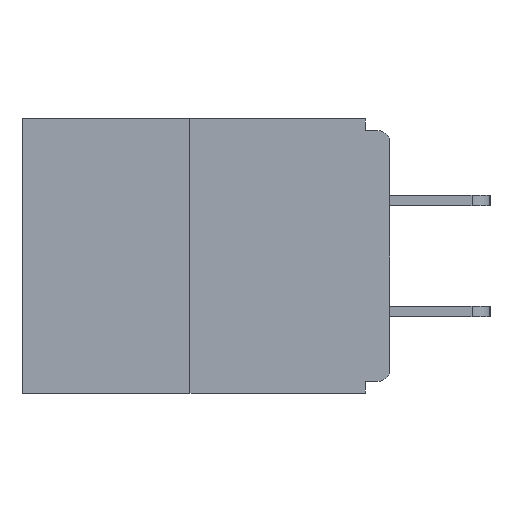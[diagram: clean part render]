
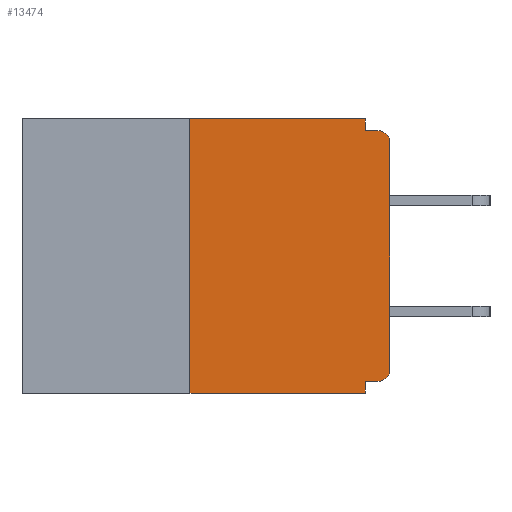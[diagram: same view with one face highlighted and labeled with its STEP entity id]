
A CAD part, left-side view. The second image highlights one B-rep face of the part: STEP entity #13474.
In plain terms, the highlighted planar face has unit normal (-1, 0, 0).
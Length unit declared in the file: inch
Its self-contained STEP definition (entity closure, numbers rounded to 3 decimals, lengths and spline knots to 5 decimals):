
#131 = CIRCLE ( 'NONE', #12091, 0.015 ) ;
#201 = VERTEX_POINT ( 'NONE', #5705 ) ;
#666 = DIRECTION ( 'NONE',  ( 0., 0., -1. ) ) ;
#750 = LINE ( 'NONE', #16430, #5694 ) ;
#1241 = CARTESIAN_POINT ( 'NONE',  ( 0., 0.031, 0. ) ) ;
#1309 = VECTOR ( 'NONE', #6027, 39.37008 ) ;
#1443 = CARTESIAN_POINT ( 'NONE',  ( 0., 0., -0.015 ) ) ;
#1554 = CARTESIAN_POINT ( 'NONE',  ( 0., 0.25, 0. ) ) ;
#1595 = ORIENTED_EDGE ( 'NONE', *, *, #3636, .F. ) ;
#1633 = EDGE_CURVE ( 'NONE', #12355, #9322, #1980, .T. ) ;
#1980 = CIRCLE ( 'NONE', #6410, 0.015 ) ;
#2694 = ORIENTED_EDGE ( 'NONE', *, *, #14655, .F. ) ;
#2749 = ORIENTED_EDGE ( 'NONE', *, *, #6295, .F. ) ;
#2947 = DIRECTION ( 'NONE',  ( 0., -1., 0. ) ) ;
#2991 = DIRECTION ( 'NONE',  ( 0., -1., 0. ) ) ;
#3419 = VERTEX_POINT ( 'NONE', #14173 ) ;
#3467 = EDGE_CURVE ( 'NONE', #9322, #201, #4333, .T. ) ;
#3636 = EDGE_CURVE ( 'NONE', #8145, #17130, #11496, .T. ) ;
#3654 = LINE ( 'NONE', #1443, #10410 ) ;
#4008 = VECTOR ( 'NONE', #2991, 39.37008 ) ;
#4129 = CARTESIAN_POINT ( 'NONE',  ( 0., 0.031, -0.015 ) ) ;
#4143 = ORIENTED_EDGE ( 'NONE', *, *, #8824, .F. ) ;
#4290 = DIRECTION ( 'NONE',  ( 0., 0., -1. ) ) ;
#4333 = LINE ( 'NONE', #5787, #8614 ) ;
#4971 = CARTESIAN_POINT ( 'NONE',  ( 0., 0.015, -0.313 ) ) ;
#5060 = CARTESIAN_POINT ( 'NONE',  ( 0., 0.015, -0.328 ) ) ;
#5574 = ORIENTED_EDGE ( 'NONE', *, *, #17512, .T. ) ;
#5694 = VECTOR ( 'NONE', #666, 39.37008 ) ;
#5705 = CARTESIAN_POINT ( 'NONE',  ( 0., 0., -0.03 ) ) ;
#5718 = VERTEX_POINT ( 'NONE', #4129 ) ;
#5787 = CARTESIAN_POINT ( 'NONE',  ( 0., 0., 0. ) ) ;
#6027 = DIRECTION ( 'NONE',  ( 0., -1., 0. ) ) ;
#6063 = CARTESIAN_POINT ( 'NONE',  ( 0., 0.25, 0. ) ) ;
#6295 = EDGE_CURVE ( 'NONE', #13297, #5718, #8324, .T. ) ;
#6410 = AXIS2_PLACEMENT_3D ( 'NONE', #4971, #13530, #13633 ) ;
#7028 = CARTESIAN_POINT ( 'NONE',  ( 0., 0.015, -0.03 ) ) ;
#7200 = VERTEX_POINT ( 'NONE', #14852 ) ;
#8093 = EDGE_CURVE ( 'NONE', #8145, #7200, #16721, .T. ) ;
#8145 = VERTEX_POINT ( 'NONE', #15782 ) ;
#8324 = LINE ( 'NONE', #1241, #17197 ) ;
#8614 = VECTOR ( 'NONE', #15790, 39.37008 ) ;
#8824 = EDGE_CURVE ( 'NONE', #17130, #13297, #17367, .T. ) ;
#8967 = CARTESIAN_POINT ( 'NONE',  ( 0., 0.015, -0.015 ) ) ;
#9135 = LINE ( 'NONE', #9775, #10214 ) ;
#9322 = VERTEX_POINT ( 'NONE', #10480 ) ;
#9775 = CARTESIAN_POINT ( 'NONE',  ( 0., 0., -0.328 ) ) ;
#10195 = CARTESIAN_POINT ( 'NONE',  ( 0., 0.46, 0. ) ) ;
#10214 = VECTOR ( 'NONE', #12315, 39.37008 ) ;
#10410 = VECTOR ( 'NONE', #2947, 39.37008 ) ;
#10480 = CARTESIAN_POINT ( 'NONE',  ( 0., 0., -0.313 ) ) ;
#10680 = DIRECTION ( 'NONE',  ( 1., 0., 0. ) ) ;
#10718 = ORIENTED_EDGE ( 'NONE', *, *, #8093, .T. ) ;
#10785 = DIRECTION ( 'NONE',  ( 0., 0., -1. ) ) ;
#11492 = CARTESIAN_POINT ( 'NONE',  ( 0., 0.46, -0.343 ) ) ;
#11496 = LINE ( 'NONE', #1554, #11742 ) ;
#11742 = VECTOR ( 'NONE', #11757, 39.37008 ) ;
#11757 = DIRECTION ( 'NONE',  ( 0., 0., 1. ) ) ;
#11811 = CARTESIAN_POINT ( 'NONE',  ( 0., 0.031, 0. ) ) ;
#12091 = AXIS2_PLACEMENT_3D ( 'NONE', #7028, #16963, #12701 ) ;
#12315 = DIRECTION ( 'NONE',  ( 0., 1., 0. ) ) ;
#12355 = VERTEX_POINT ( 'NONE', #5060 ) ;
#12701 = DIRECTION ( 'NONE',  ( 0., 0., -1. ) ) ;
#12763 = ORIENTED_EDGE ( 'NONE', *, *, #17640, .F. ) ;
#13059 = ORIENTED_EDGE ( 'NONE', *, *, #1633, .T. ) ;
#13297 = VERTEX_POINT ( 'NONE', #11811 ) ;
#13372 = VERTEX_POINT ( 'NONE', #8967 ) ;
#13474 = ADVANCED_FACE ( 'NONE', ( #13569 ), #15072, .F. ) ;
#13530 = DIRECTION ( 'NONE',  ( -1., 0., 0. ) ) ;
#13569 = FACE_OUTER_BOUND ( 'NONE', #15793, .T. ) ;
#13633 = DIRECTION ( 'NONE',  ( 0., 0., -1. ) ) ;
#14073 = ORIENTED_EDGE ( 'NONE', *, *, #18419, .F. ) ;
#14173 = CARTESIAN_POINT ( 'NONE',  ( 0., 0.031, -0.328 ) ) ;
#14655 = EDGE_CURVE ( 'NONE', #12355, #3419, #9135, .T. ) ;
#14852 = CARTESIAN_POINT ( 'NONE',  ( 0., 0.031, -0.343 ) ) ;
#14889 = AXIS2_PLACEMENT_3D ( 'NONE', #14951, #10680, #10785 ) ;
#14951 = CARTESIAN_POINT ( 'NONE',  ( 0., 0.46, 0. ) ) ;
#15072 = PLANE ( 'NONE',  #14889 ) ;
#15782 = CARTESIAN_POINT ( 'NONE',  ( 0., 0.25, -0.343 ) ) ;
#15790 = DIRECTION ( 'NONE',  ( 0., 0., 1. ) ) ;
#15793 = EDGE_LOOP ( 'NONE', ( #4143, #1595, #10718, #14073, #2694, #13059, #16270, #5574, #12763, #2749 ) ) ;
#16270 = ORIENTED_EDGE ( 'NONE', *, *, #3467, .T. ) ;
#16430 = CARTESIAN_POINT ( 'NONE',  ( 0., 0.031, -0.343 ) ) ;
#16721 = LINE ( 'NONE', #11492, #4008 ) ;
#16963 = DIRECTION ( 'NONE',  ( -1., 0., 0. ) ) ;
#17130 = VERTEX_POINT ( 'NONE', #6063 ) ;
#17197 = VECTOR ( 'NONE', #4290, 39.37008 ) ;
#17367 = LINE ( 'NONE', #10195, #1309 ) ;
#17512 = EDGE_CURVE ( 'NONE', #201, #13372, #131, .T. ) ;
#17640 = EDGE_CURVE ( 'NONE', #5718, #13372, #3654, .T. ) ;
#18419 = EDGE_CURVE ( 'NONE', #3419, #7200, #750, .T. ) ;
